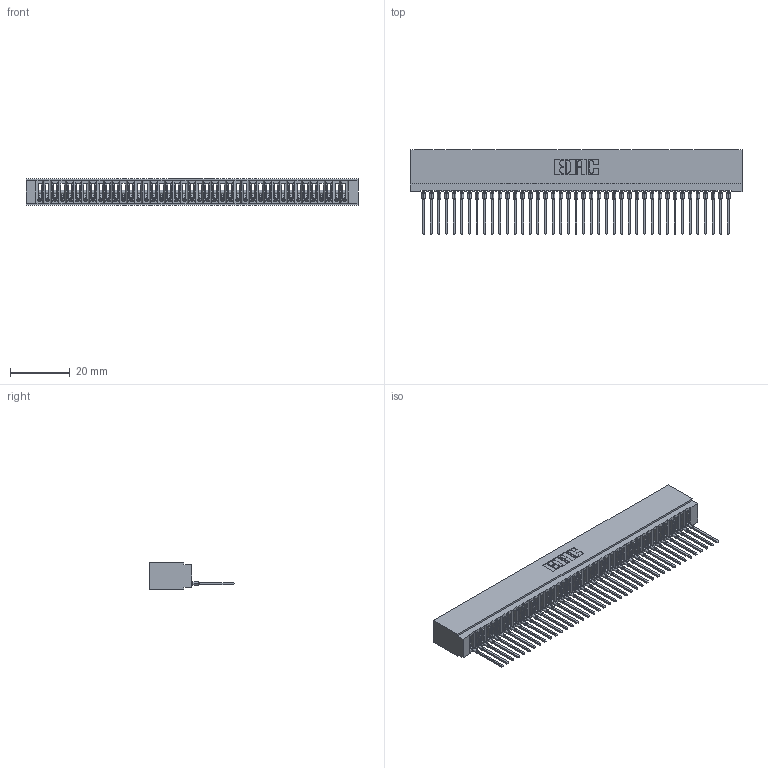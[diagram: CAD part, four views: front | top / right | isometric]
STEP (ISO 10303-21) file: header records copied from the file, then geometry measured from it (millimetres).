
FILE_DESCRIPTION (( 'STEP AP203' ), '1' );
FILE_NAME ('725-041-545-101.STEP', '2026-03-05T22:38:18', ( '' ), ( '' ), 'SwSTEP 2.0', 'SolidWorks 2023', '' );
FILE_SCHEMA (( 'CONFIG_CONTROL_DESIGN' ));
Length unit declared in the file: millimetre
Products named in the file (3): 725-041-545-101; 725 Part_Insulator Option - 01; 745-292-001_545
Assembly tree (42 placements, depth 2):
  725-041-545-101
    725 Part_Insulator Option - 01
    745-292-001_545  x41
Bounding box: 110.74 x 28.21 x 8.89 mm (x, y, z)
Volume: 8529.6 mm3; surface area: 17000 mm2
Topology: 42 solids, 42 shells, 4687 faces, 12882 edges, 8122 vertices
Faces by surface type: plane 2802, bspline 820, cylinder 819, torus 246
Entity records: 67813 total; most frequent: CARTESIAN_POINT 12450, ORIENTED_EDGE 11924, DIRECTION 10338, EDGE_CURVE 5962, LINE 5534, VECTOR 5534, VERTEX_POINT 3802, AXIS2_PLACEMENT_3D 2402
